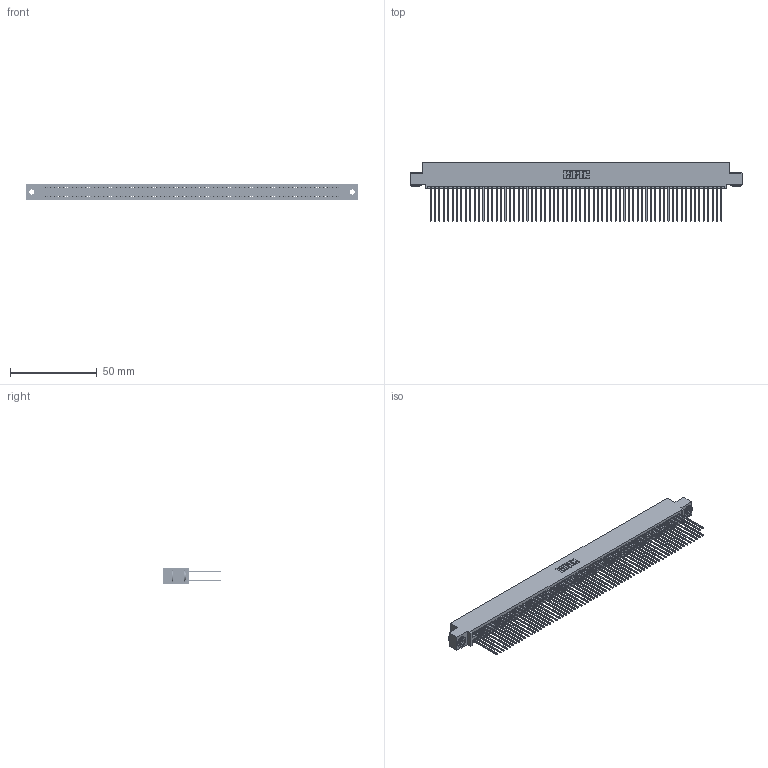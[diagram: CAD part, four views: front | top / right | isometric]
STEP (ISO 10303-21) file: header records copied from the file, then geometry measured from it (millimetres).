
FILE_DESCRIPTION (( 'STEP AP203' ), '1' );
FILE_NAME ('345-134-541-503.STEP', '2018-10-20T09:22:23', ( '' ), ( '' ), 'SwSTEP 2.0', 'SolidWorks 2016', '' );
FILE_SCHEMA (( 'CONFIG_CONTROL_DESIGN' ));
Length unit declared in the file: inch
Products named in the file (4): 345-134-541-503; 345 Part_0.110 Offset - 0.156 Dia-TH; 345-250-002_345-250-002-102; 345-292-001_345-293-141
Assembly tree (137 placements, depth 2):
  345-134-541-503
    345 Part_0.110 Offset - 0.156 Dia-TH
    345-292-001_345-293-141  x134
    345-250-002_345-250-002-102  x2
Bounding box: 191.39 x 33.96 x 9.4 mm (x, y, z)
Volume: 19538.6 mm3; surface area: 33277.1 mm2
Topology: 137 solids, 137 shells, 6868 faces, 20395 edges, 13414 vertices
Faces by surface type: plane 4516, cylinder 2344, cone 8
Entity records: 50004 total; most frequent: CARTESIAN_POINT 8335, ORIENTED_EDGE 8262, DIRECTION 7349, EDGE_CURVE 4131, VECTOR 3707, LINE 3707, VERTEX_POINT 2750, AXIS2_PLACEMENT_3D 1821
